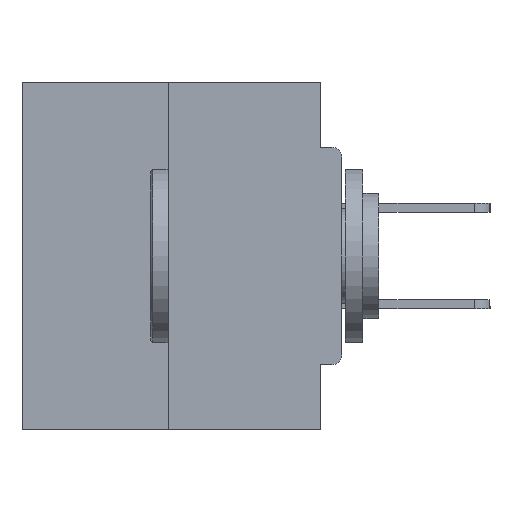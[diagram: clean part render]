
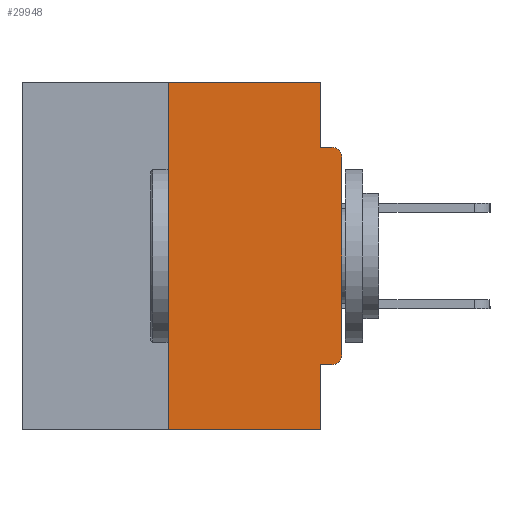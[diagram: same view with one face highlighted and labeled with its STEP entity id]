
A CAD part, left-side view. The second image highlights one B-rep face of the part: STEP entity #29948.
In plain terms, the highlighted planar face has unit normal (-1, 0, 0).
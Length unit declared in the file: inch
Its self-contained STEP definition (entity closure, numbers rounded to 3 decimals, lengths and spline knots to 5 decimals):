
#354 = CARTESIAN_POINT ( 'NONE',  ( 0., 0.031, 0. ) ) ;
#629 = DIRECTION ( 'NONE',  ( 1., 0., 0. ) ) ;
#1559 = EDGE_CURVE ( 'NONE', #29147, #19920, #1889, .T. ) ;
#1889 = LINE ( 'NONE', #7279, #15774 ) ;
#1944 = ORIENTED_EDGE ( 'NONE', *, *, #7882, .F. ) ;
#1958 = CARTESIAN_POINT ( 'NONE',  ( 0., 0.015, -0.1085 ) ) ;
#2632 = CARTESIAN_POINT ( 'NONE',  ( 0., 0., -0.4065 ) ) ;
#2652 = EDGE_LOOP ( 'NONE', ( #4617, #15518, #18876, #27533, #11199, #6739, #27027, #11646, #14993, #1944 ) ) ;
#3589 = DIRECTION ( 'NONE',  ( 0., 1., 0. ) ) ;
#4145 = LINE ( 'NONE', #22251, #31098 ) ;
#4601 = EDGE_CURVE ( 'NONE', #31093, #16197, #4145, .T. ) ;
#4617 = ORIENTED_EDGE ( 'NONE', *, *, #19662, .F. ) ;
#5153 = VECTOR ( 'NONE', #30443, 39.37008 ) ;
#5186 = EDGE_CURVE ( 'NONE', #27570, #31093, #26181, .T. ) ;
#5593 = CARTESIAN_POINT ( 'NONE',  ( 0., 0.031, -0.5 ) ) ;
#5747 = EDGE_CURVE ( 'NONE', #13936, #24949, #27650, .T. ) ;
#6578 = CARTESIAN_POINT ( 'NONE',  ( 0., 0.25, 0. ) ) ;
#6739 = ORIENTED_EDGE ( 'NONE', *, *, #27286, .T. ) ;
#6895 = CARTESIAN_POINT ( 'NONE',  ( 0., 0., -0.3915 ) ) ;
#6985 = DIRECTION ( 'NONE',  ( 0., 0., -1. ) ) ;
#7279 = CARTESIAN_POINT ( 'NONE',  ( 0., 0., -0.0935 ) ) ;
#7882 = EDGE_CURVE ( 'NONE', #15549, #29147, #18462, .T. ) ;
#8773 = PLANE ( 'NONE',  #14539 ) ;
#9300 = CIRCLE ( 'NONE', #21473, 0.015 ) ;
#9422 = VECTOR ( 'NONE', #22083, 39.37008 ) ;
#10291 = VECTOR ( 'NONE', #31031, 39.37008 ) ;
#10341 = AXIS2_PLACEMENT_3D ( 'NONE', #1958, #33285, #25810 ) ;
#11199 = ORIENTED_EDGE ( 'NONE', *, *, #5186, .F. ) ;
#11382 = DIRECTION ( 'NONE',  ( 0., 0., -1. ) ) ;
#11646 = ORIENTED_EDGE ( 'NONE', *, *, #11659, .T. ) ;
#11659 = EDGE_CURVE ( 'NONE', #24949, #19920, #16188, .T. ) ;
#12183 = CARTESIAN_POINT ( 'NONE',  ( 0., 0.46, 0. ) ) ;
#12605 = DIRECTION ( 'NONE',  ( -1., 0., 0. ) ) ;
#12723 = CARTESIAN_POINT ( 'NONE',  ( 0., 0.46, -0.5 ) ) ;
#12753 = EDGE_CURVE ( 'NONE', #27224, #16173, #14722, .T. ) ;
#13257 = CARTESIAN_POINT ( 'NONE',  ( 0., 0.031, -0.4065 ) ) ;
#13748 = VECTOR ( 'NONE', #19922, 39.37008 ) ;
#13936 = VERTEX_POINT ( 'NONE', #6895 ) ;
#14539 = AXIS2_PLACEMENT_3D ( 'NONE', #29446, #629, #11382 ) ;
#14722 = LINE ( 'NONE', #6578, #9422 ) ;
#14993 = ORIENTED_EDGE ( 'NONE', *, *, #1559, .F. ) ;
#15238 = DIRECTION ( 'NONE',  ( 0., 0., -1. ) ) ;
#15518 = ORIENTED_EDGE ( 'NONE', *, *, #12753, .F. ) ;
#15549 = VERTEX_POINT ( 'NONE', #354 ) ;
#15774 = VECTOR ( 'NONE', #30797, 39.37008 ) ;
#16068 = FACE_OUTER_BOUND ( 'NONE', #2652, .T. ) ;
#16086 = CARTESIAN_POINT ( 'NONE',  ( 0., 0.25, 0. ) ) ;
#16173 = VERTEX_POINT ( 'NONE', #16086 ) ;
#16188 = CIRCLE ( 'NONE', #10341, 0.015 ) ;
#16197 = VERTEX_POINT ( 'NONE', #5593 ) ;
#16969 = CARTESIAN_POINT ( 'NONE',  ( 0., 0., 0. ) ) ;
#17007 = LINE ( 'NONE', #12723, #32595 ) ;
#18462 = LINE ( 'NONE', #30697, #10291 ) ;
#18876 = ORIENTED_EDGE ( 'NONE', *, *, #28381, .T. ) ;
#19662 = EDGE_CURVE ( 'NONE', #16173, #15549, #28838, .T. ) ;
#19920 = VERTEX_POINT ( 'NONE', #31716 ) ;
#19922 = DIRECTION ( 'NONE',  ( 0., 0., 1. ) ) ;
#20597 = DIRECTION ( 'NONE',  ( 0., -1., 0. ) ) ;
#21473 = AXIS2_PLACEMENT_3D ( 'NONE', #30783, #12605, #15238 ) ;
#22083 = DIRECTION ( 'NONE',  ( 0., 0., 1. ) ) ;
#22251 = CARTESIAN_POINT ( 'NONE',  ( 0., 0.031, -0.5 ) ) ;
#22645 = CARTESIAN_POINT ( 'NONE',  ( 0., 0.25, -0.5 ) ) ;
#23783 = CARTESIAN_POINT ( 'NONE',  ( 0., 0.015, -0.4065 ) ) ;
#24949 = VERTEX_POINT ( 'NONE', #31697 ) ;
#25810 = DIRECTION ( 'NONE',  ( 0., 0., -1. ) ) ;
#26181 = LINE ( 'NONE', #2632, #32314 ) ;
#27027 = ORIENTED_EDGE ( 'NONE', *, *, #5747, .T. ) ;
#27224 = VERTEX_POINT ( 'NONE', #22645 ) ;
#27286 = EDGE_CURVE ( 'NONE', #27570, #13936, #9300, .T. ) ;
#27533 = ORIENTED_EDGE ( 'NONE', *, *, #4601, .F. ) ;
#27570 = VERTEX_POINT ( 'NONE', #23783 ) ;
#27650 = LINE ( 'NONE', #16969, #13748 ) ;
#28381 = EDGE_CURVE ( 'NONE', #27224, #16197, #17007, .T. ) ;
#28838 = LINE ( 'NONE', #12183, #5153 ) ;
#29147 = VERTEX_POINT ( 'NONE', #30857 ) ;
#29446 = CARTESIAN_POINT ( 'NONE',  ( 0., 0.46, 0. ) ) ;
#29948 = ADVANCED_FACE ( 'NONE', ( #16068 ), #8773, .F. ) ;
#30443 = DIRECTION ( 'NONE',  ( 0., -1., 0. ) ) ;
#30697 = CARTESIAN_POINT ( 'NONE',  ( 0., 0.031, 0. ) ) ;
#30783 = CARTESIAN_POINT ( 'NONE',  ( 0., 0.015, -0.3915 ) ) ;
#30797 = DIRECTION ( 'NONE',  ( 0., -1., 0. ) ) ;
#30857 = CARTESIAN_POINT ( 'NONE',  ( 0., 0.031, -0.0935 ) ) ;
#31031 = DIRECTION ( 'NONE',  ( 0., 0., -1. ) ) ;
#31093 = VERTEX_POINT ( 'NONE', #13257 ) ;
#31098 = VECTOR ( 'NONE', #6985, 39.37008 ) ;
#31697 = CARTESIAN_POINT ( 'NONE',  ( 0., 0., -0.1085 ) ) ;
#31716 = CARTESIAN_POINT ( 'NONE',  ( 0., 0.015, -0.0935 ) ) ;
#32314 = VECTOR ( 'NONE', #3589, 39.37008 ) ;
#32595 = VECTOR ( 'NONE', #20597, 39.37008 ) ;
#33285 = DIRECTION ( 'NONE',  ( -1., 0., 0. ) ) ;
